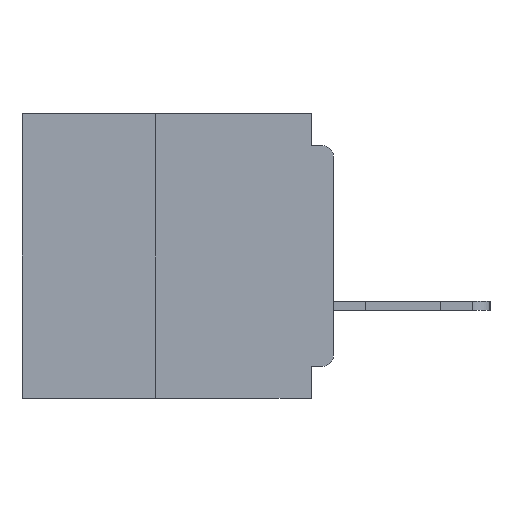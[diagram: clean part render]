
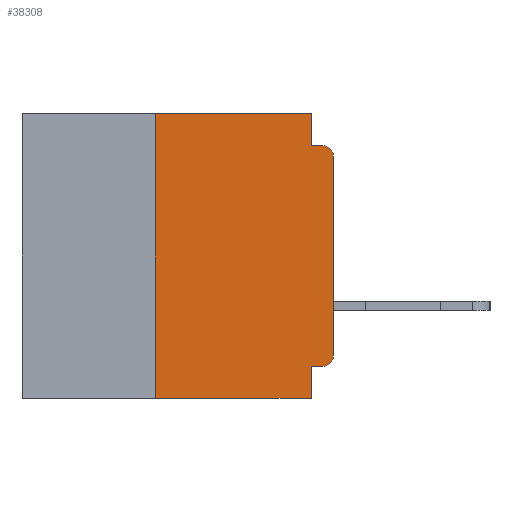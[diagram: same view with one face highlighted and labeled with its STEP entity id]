
A CAD part, left-side view. The second image highlights one B-rep face of the part: STEP entity #38308.
In plain terms, the highlighted planar face has unit normal (-1, 0, 0).
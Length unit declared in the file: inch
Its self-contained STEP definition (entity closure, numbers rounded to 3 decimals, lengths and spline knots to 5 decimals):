
#208 = EDGE_CURVE ( 'NONE', #34055, #2421, #16039, .T. ) ;
#231 = CARTESIAN_POINT ( 'NONE',  ( 0., 0., -0.06 ) ) ;
#384 = CIRCLE ( 'NONE', #26087, 0.015 ) ;
#932 = VERTEX_POINT ( 'NONE', #231 ) ;
#2382 = ORIENTED_EDGE ( 'NONE', *, *, #4956, .F. ) ;
#2421 = VERTEX_POINT ( 'NONE', #20070 ) ;
#2495 = VECTOR ( 'NONE', #46096, 39.37008 ) ;
#3354 = VECTOR ( 'NONE', #26808, 39.37008 ) ;
#3522 = DIRECTION ( 'NONE',  ( 0., 0., -1. ) ) ;
#3935 = LINE ( 'NONE', #6049, #21050 ) ;
#4053 = VECTOR ( 'NONE', #9940, 39.37008 ) ;
#4418 = LINE ( 'NONE', #13600, #40373 ) ;
#4956 = EDGE_CURVE ( 'NONE', #24472, #39816, #19636, .T. ) ;
#6049 = CARTESIAN_POINT ( 'NONE',  ( 0., 0.031, -0.4 ) ) ;
#6909 = CARTESIAN_POINT ( 'NONE',  ( 0., 0., -0.355 ) ) ;
#6993 = EDGE_CURVE ( 'NONE', #31239, #24800, #3935, .T. ) ;
#9758 = CARTESIAN_POINT ( 'NONE',  ( 0., 0.015, -0.045 ) ) ;
#9940 = DIRECTION ( 'NONE',  ( 0., 0., 1. ) ) ;
#13387 = ORIENTED_EDGE ( 'NONE', *, *, #38151, .T. ) ;
#13600 = CARTESIAN_POINT ( 'NONE',  ( 0., 0.437, 0. ) ) ;
#14484 = EDGE_CURVE ( 'NONE', #32325, #43012, #26046, .T. ) ;
#14816 = PLANE ( 'NONE',  #24378 ) ;
#14818 = CARTESIAN_POINT ( 'NONE',  ( 0., 0.031, 0. ) ) ;
#15181 = VERTEX_POINT ( 'NONE', #9758 ) ;
#15751 = EDGE_CURVE ( 'NONE', #932, #15181, #384, .T. ) ;
#15791 = CARTESIAN_POINT ( 'NONE',  ( 0., 0.437, -0.4 ) ) ;
#16039 = LINE ( 'NONE', #45306, #4053 ) ;
#17389 = CARTESIAN_POINT ( 'NONE',  ( 0., 0., -0.34 ) ) ;
#18214 = ORIENTED_EDGE ( 'NONE', *, *, #45654, .F. ) ;
#18238 = LINE ( 'NONE', #6909, #27762 ) ;
#18494 = DIRECTION ( 'NONE',  ( 1., 0., 0. ) ) ;
#19085 = CARTESIAN_POINT ( 'NONE',  ( 0., 0., -0.045 ) ) ;
#19216 = CARTESIAN_POINT ( 'NONE',  ( 0., 0.031, -0.045 ) ) ;
#19636 = LINE ( 'NONE', #14818, #28000 ) ;
#20026 = VECTOR ( 'NONE', #43910, 39.37008 ) ;
#20070 = CARTESIAN_POINT ( 'NONE',  ( 0., 0.25, 0. ) ) ;
#20332 = DIRECTION ( 'NONE',  ( -1., 0., 0. ) ) ;
#21050 = VECTOR ( 'NONE', #27553, 39.37008 ) ;
#23006 = LINE ( 'NONE', #24929, #2495 ) ;
#23465 = ORIENTED_EDGE ( 'NONE', *, *, #43812, .F. ) ;
#24378 = AXIS2_PLACEMENT_3D ( 'NONE', #39801, #18494, #43351 ) ;
#24472 = VERTEX_POINT ( 'NONE', #42753 ) ;
#24800 = VERTEX_POINT ( 'NONE', #27271 ) ;
#24929 = CARTESIAN_POINT ( 'NONE',  ( 0., 0., 0. ) ) ;
#25261 = DIRECTION ( 'NONE',  ( -1., 0., 0. ) ) ;
#25630 = CARTESIAN_POINT ( 'NONE',  ( 0., 0.25, -0.4 ) ) ;
#26046 = CIRCLE ( 'NONE', #45445, 0.015 ) ;
#26087 = AXIS2_PLACEMENT_3D ( 'NONE', #46420, #25261, #3522 ) ;
#26808 = DIRECTION ( 'NONE',  ( 0., -1., 0. ) ) ;
#27171 = CARTESIAN_POINT ( 'NONE',  ( 0., 0.031, -0.355 ) ) ;
#27271 = CARTESIAN_POINT ( 'NONE',  ( 0., 0.031, -0.4 ) ) ;
#27429 = EDGE_LOOP ( 'NONE', ( #13387, #30212, #23465, #2382, #18214, #44760, #36239, #38177, #39238, #44379 ) ) ;
#27553 = DIRECTION ( 'NONE',  ( 0., 0., -1. ) ) ;
#27762 = VECTOR ( 'NONE', #32109, 39.37008 ) ;
#28000 = VECTOR ( 'NONE', #29292, 39.37008 ) ;
#29292 = DIRECTION ( 'NONE',  ( 0., 0., -1. ) ) ;
#29507 = LINE ( 'NONE', #19085, #20026 ) ;
#30212 = ORIENTED_EDGE ( 'NONE', *, *, #15751, .T. ) ;
#31239 = VERTEX_POINT ( 'NONE', #27171 ) ;
#32109 = DIRECTION ( 'NONE',  ( 0., 1., 0. ) ) ;
#32159 = LINE ( 'NONE', #15791, #3354 ) ;
#32325 = VERTEX_POINT ( 'NONE', #44057 ) ;
#34055 = VERTEX_POINT ( 'NONE', #25630 ) ;
#36239 = ORIENTED_EDGE ( 'NONE', *, *, #44802, .T. ) ;
#38151 = EDGE_CURVE ( 'NONE', #43012, #932, #23006, .T. ) ;
#38177 = ORIENTED_EDGE ( 'NONE', *, *, #6993, .F. ) ;
#38308 = ADVANCED_FACE ( 'NONE', ( #43461 ), #14816, .F. ) ;
#39238 = ORIENTED_EDGE ( 'NONE', *, *, #44530, .F. ) ;
#39801 = CARTESIAN_POINT ( 'NONE',  ( 0., 0.437, 0. ) ) ;
#39816 = VERTEX_POINT ( 'NONE', #19216 ) ;
#40373 = VECTOR ( 'NONE', #42178, 39.37008 ) ;
#41553 = CARTESIAN_POINT ( 'NONE',  ( 0., 0.015, -0.34 ) ) ;
#42178 = DIRECTION ( 'NONE',  ( 0., -1., 0. ) ) ;
#42753 = CARTESIAN_POINT ( 'NONE',  ( 0., 0.031, 0. ) ) ;
#43012 = VERTEX_POINT ( 'NONE', #17389 ) ;
#43351 = DIRECTION ( 'NONE',  ( 0., 0., -1. ) ) ;
#43461 = FACE_OUTER_BOUND ( 'NONE', #27429, .T. ) ;
#43812 = EDGE_CURVE ( 'NONE', #39816, #15181, #29507, .T. ) ;
#43910 = DIRECTION ( 'NONE',  ( 0., -1., 0. ) ) ;
#44057 = CARTESIAN_POINT ( 'NONE',  ( 0., 0.015, -0.355 ) ) ;
#44379 = ORIENTED_EDGE ( 'NONE', *, *, #14484, .T. ) ;
#44530 = EDGE_CURVE ( 'NONE', #32325, #31239, #18238, .T. ) ;
#44760 = ORIENTED_EDGE ( 'NONE', *, *, #208, .F. ) ;
#44802 = EDGE_CURVE ( 'NONE', #34055, #24800, #32159, .T. ) ;
#45092 = DIRECTION ( 'NONE',  ( 0., 0., -1. ) ) ;
#45306 = CARTESIAN_POINT ( 'NONE',  ( 0., 0.25, -0.4 ) ) ;
#45445 = AXIS2_PLACEMENT_3D ( 'NONE', #41553, #20332, #45092 ) ;
#45654 = EDGE_CURVE ( 'NONE', #2421, #24472, #4418, .T. ) ;
#46096 = DIRECTION ( 'NONE',  ( 0., 0., 1. ) ) ;
#46420 = CARTESIAN_POINT ( 'NONE',  ( 0., 0.015, -0.06 ) ) ;
